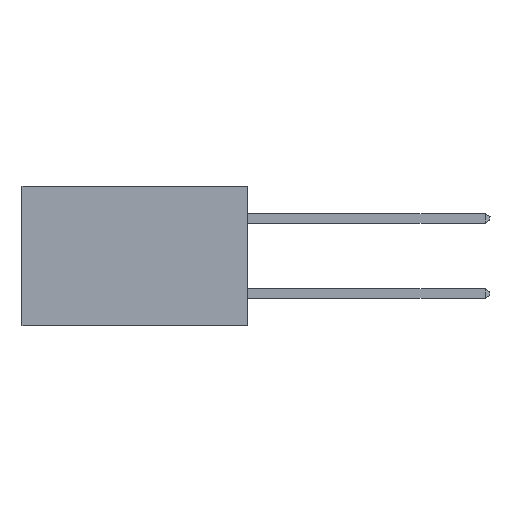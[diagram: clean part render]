
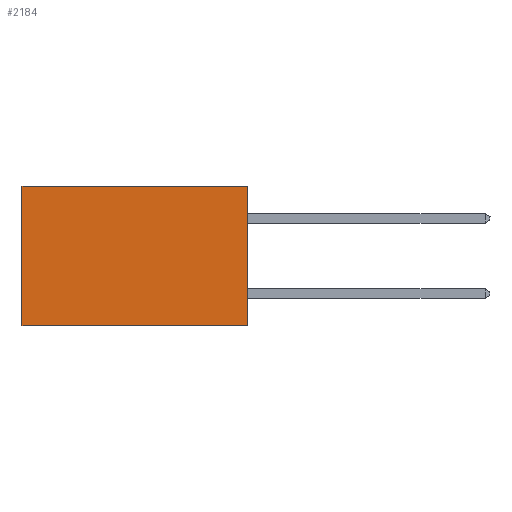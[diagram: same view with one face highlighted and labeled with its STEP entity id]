
A CAD part, left-side view. The second image highlights one B-rep face of the part: STEP entity #2184.
In plain terms, the highlighted planar face has unit normal (-1, 0, 0).
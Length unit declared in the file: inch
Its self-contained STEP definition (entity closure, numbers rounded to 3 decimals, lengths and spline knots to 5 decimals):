
#1494 = CARTESIAN_POINT ( 'NONE',  ( 0.298, 0., 0. ) ) ;
#1559 = DIRECTION ( 'NONE',  ( 1., 0., 0. ) ) ;
#2184 = ADVANCED_FACE ( 'NONE', ( #11346 ), #11450, .F. ) ;
#2563 = VERTEX_POINT ( 'NONE', #13977 ) ;
#2875 = AXIS2_PLACEMENT_3D ( 'NONE', #9062, #1559, #10471 ) ;
#4400 = VECTOR ( 'NONE', #8529, 39.37008 ) ;
#4404 = EDGE_CURVE ( 'NONE', #2563, #13008, #7703, .T. ) ;
#4730 = EDGE_CURVE ( 'NONE', #7129, #13008, #4989, .T. ) ;
#4747 = CARTESIAN_POINT ( 'NONE',  ( 0.298, 0.6, 0. ) ) ;
#4989 = LINE ( 'NONE', #12316, #15906 ) ;
#5017 = VECTOR ( 'NONE', #12878, 39.37008 ) ;
#5431 = LINE ( 'NONE', #10470, #5017 ) ;
#5963 = ORIENTED_EDGE ( 'NONE', *, *, #4404, .T. ) ;
#6075 = ORIENTED_EDGE ( 'NONE', *, *, #4730, .F. ) ;
#7129 = VERTEX_POINT ( 'NONE', #11572 ) ;
#7191 = CARTESIAN_POINT ( 'NONE',  ( 0.298, 0.6, -0.37 ) ) ;
#7615 = DIRECTION ( 'NONE',  ( 0., 0., -1. ) ) ;
#7703 = LINE ( 'NONE', #4747, #4400 ) ;
#7982 = ORIENTED_EDGE ( 'NONE', *, *, #12260, .T. ) ;
#8387 = VECTOR ( 'NONE', #7615, 39.37008 ) ;
#8529 = DIRECTION ( 'NONE',  ( 0., 0., -1. ) ) ;
#9062 = CARTESIAN_POINT ( 'NONE',  ( 0.298, 0., 0. ) ) ;
#9506 = EDGE_LOOP ( 'NONE', ( #5963, #6075, #10225, #7982 ) ) ;
#9937 = EDGE_CURVE ( 'NONE', #15392, #7129, #15441, .T. ) ;
#10225 = ORIENTED_EDGE ( 'NONE', *, *, #9937, .F. ) ;
#10470 = CARTESIAN_POINT ( 'NONE',  ( 0.298, 0., 0. ) ) ;
#10471 = DIRECTION ( 'NONE',  ( 0., 0., -1. ) ) ;
#11346 = FACE_OUTER_BOUND ( 'NONE', #9506, .T. ) ;
#11450 = PLANE ( 'NONE',  #2875 ) ;
#11572 = CARTESIAN_POINT ( 'NONE',  ( 0.298, 0., -0.37 ) ) ;
#12260 = EDGE_CURVE ( 'NONE', #15392, #2563, #5431, .T. ) ;
#12316 = CARTESIAN_POINT ( 'NONE',  ( 0.298, 0., -0.37 ) ) ;
#12878 = DIRECTION ( 'NONE',  ( 0., 1., 0. ) ) ;
#13008 = VERTEX_POINT ( 'NONE', #7191 ) ;
#13743 = CARTESIAN_POINT ( 'NONE',  ( 0.298, 0., 0. ) ) ;
#13977 = CARTESIAN_POINT ( 'NONE',  ( 0.298, 0.6, 0. ) ) ;
#14861 = DIRECTION ( 'NONE',  ( 0., 1., 0. ) ) ;
#15392 = VERTEX_POINT ( 'NONE', #1494 ) ;
#15441 = LINE ( 'NONE', #13743, #8387 ) ;
#15906 = VECTOR ( 'NONE', #14861, 39.37008 ) ;
